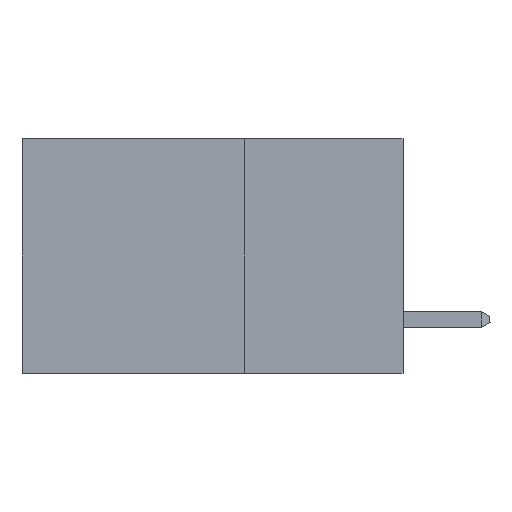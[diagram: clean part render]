
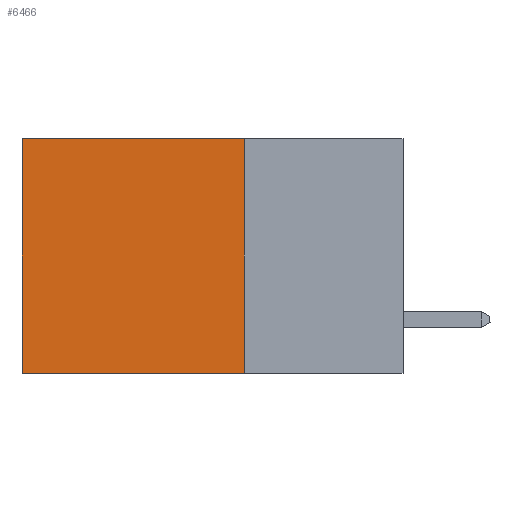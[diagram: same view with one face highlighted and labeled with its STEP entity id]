
A CAD part, left-side view. The second image highlights one B-rep face of the part: STEP entity #6466.
In plain terms, the highlighted planar face has unit normal (-1, 0, 0).
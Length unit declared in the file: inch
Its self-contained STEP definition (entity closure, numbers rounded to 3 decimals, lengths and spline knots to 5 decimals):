
#487 = LINE ( 'NONE', #1503, #9905 ) ;
#813 = EDGE_CURVE ( 'NONE', #7329, #5846, #487, .T. ) ;
#1119 = DIRECTION ( 'NONE',  ( 0., 0., -1. ) ) ;
#1325 = CARTESIAN_POINT ( 'NONE',  ( 0.2875, 0.25, 0. ) ) ;
#1503 = CARTESIAN_POINT ( 'NONE',  ( 0.2875, 0.25, 0. ) ) ;
#1664 = LINE ( 'NONE', #6307, #11659 ) ;
#2741 = DIRECTION ( 'NONE',  ( 0., 0., -1. ) ) ;
#3036 = EDGE_CURVE ( 'NONE', #7329, #4947, #8280, .T. ) ;
#3413 = LINE ( 'NONE', #11665, #8270 ) ;
#3481 = DIRECTION ( 'NONE',  ( 0., 1., 0. ) ) ;
#3929 = VERTEX_POINT ( 'NONE', #6390 ) ;
#3970 = EDGE_CURVE ( 'NONE', #5846, #3929, #1664, .T. ) ;
#4467 = ORIENTED_EDGE ( 'NONE', *, *, #813, .T. ) ;
#4947 = VERTEX_POINT ( 'NONE', #9396 ) ;
#5722 = PLANE ( 'NONE',  #10947 ) ;
#5765 = DIRECTION ( 'NONE',  ( 1., 0., 0. ) ) ;
#5846 = VERTEX_POINT ( 'NONE', #9165 ) ;
#5892 = DIRECTION ( 'NONE',  ( 0., 0., -1. ) ) ;
#6230 = DIRECTION ( 'NONE',  ( 0., 1., 0. ) ) ;
#6307 = CARTESIAN_POINT ( 'NONE',  ( 0.2875, 0.6, 0. ) ) ;
#6390 = CARTESIAN_POINT ( 'NONE',  ( 0.2875, 0.6, -0.37 ) ) ;
#6466 = ADVANCED_FACE ( 'NONE', ( #6795 ), #5722, .F. ) ;
#6591 = VECTOR ( 'NONE', #5892, 39.37008 ) ;
#6795 = FACE_OUTER_BOUND ( 'NONE', #11076, .T. ) ;
#7329 = VERTEX_POINT ( 'NONE', #1325 ) ;
#8270 = VECTOR ( 'NONE', #6230, 39.37008 ) ;
#8280 = LINE ( 'NONE', #8544, #6591 ) ;
#8544 = CARTESIAN_POINT ( 'NONE',  ( 0.2875, 0.25, 0. ) ) ;
#9165 = CARTESIAN_POINT ( 'NONE',  ( 0.2875, 0.6, 0. ) ) ;
#9396 = CARTESIAN_POINT ( 'NONE',  ( 0.2875, 0.25, -0.37 ) ) ;
#9502 = ORIENTED_EDGE ( 'NONE', *, *, #3970, .T. ) ;
#9905 = VECTOR ( 'NONE', #3481, 39.37008 ) ;
#10210 = ORIENTED_EDGE ( 'NONE', *, *, #3036, .F. ) ;
#10335 = CARTESIAN_POINT ( 'NONE',  ( 0.2875, 0.25, 0. ) ) ;
#10947 = AXIS2_PLACEMENT_3D ( 'NONE', #10335, #5765, #1119 ) ;
#11041 = ORIENTED_EDGE ( 'NONE', *, *, #11574, .F. ) ;
#11076 = EDGE_LOOP ( 'NONE', ( #9502, #11041, #10210, #4467 ) ) ;
#11574 = EDGE_CURVE ( 'NONE', #4947, #3929, #3413, .T. ) ;
#11659 = VECTOR ( 'NONE', #2741, 39.37008 ) ;
#11665 = CARTESIAN_POINT ( 'NONE',  ( 0.2875, 0.25, -0.37 ) ) ;
